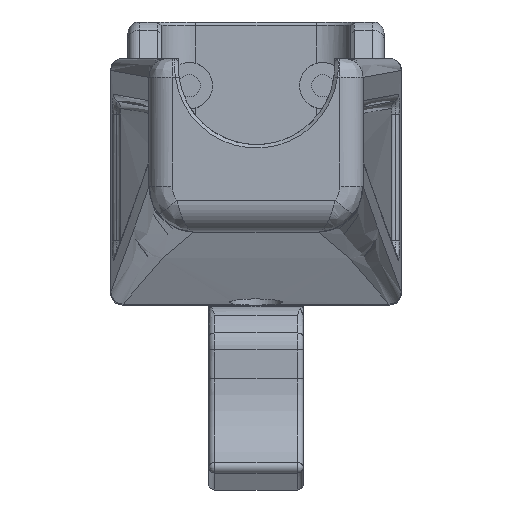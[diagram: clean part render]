
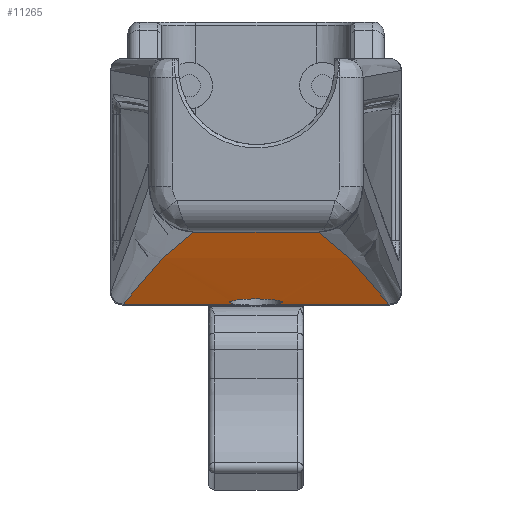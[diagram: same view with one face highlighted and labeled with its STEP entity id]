
A CAD part, front view. The second image highlights one B-rep face of the part: STEP entity #11265.
In plain terms, the highlighted cylindrical face has radius 1594.73 mm (diameter 3189.46 mm), a partial arc.
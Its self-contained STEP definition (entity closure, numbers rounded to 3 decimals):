
#330=B_SPLINE_CURVE_WITH_KNOTS('',3,(#18662,#18663,#18664,#18665,#18666,
#18667,#18668,#18669,#18670,#18671,#18672,#18673,#18674,#18675,#18676,#18677,
#18678,#18679,#18680,#18681,#18682,#18683,#18684),.UNSPECIFIED.,.F.,.F.,
(4,2,2,2,2,2,3,2,2,2,4),(-0.946,-0.852,-0.681,
-0.51,-0.339,-0.169,0.,0.17,
0.34,0.51,0.681),.UNSPECIFIED.);
#332=B_SPLINE_CURVE_WITH_KNOTS('',3,(#18700,#18701,#18702,#18703,#18704,
#18705),.UNSPECIFIED.,.F.,.F.,(4,2,4),(0.681,0.851,
0.946),.UNSPECIFIED.);
#459=B_SPLINE_CURVE_WITH_KNOTS('',3,(#21532,#21533,#21534,#21535),
 .UNSPECIFIED.,.F.,.F.,(4,4),(-0.316,-0.304),
 .UNSPECIFIED.);
#462=B_SPLINE_CURVE_WITH_KNOTS('',3,(#22020,#22021,#22022,#22023),
 .UNSPECIFIED.,.F.,.F.,(4,4),(-15.111,-0.316),
 .UNSPECIFIED.);
#472=B_SPLINE_CURVE_WITH_KNOTS('',3,(#22319,#22320,#22321,#22322),
 .UNSPECIFIED.,.F.,.F.,(4,4),(-0.316,-0.304),
 .UNSPECIFIED.);
#477=B_SPLINE_CURVE_WITH_KNOTS('',3,(#22797,#22798,#22799,#22800),
 .UNSPECIFIED.,.F.,.F.,(4,4),(-15.111,-0.316),
 .UNSPECIFIED.);
#1774=FACE_OUTER_BOUND('',#2480,.T.);
#2480=EDGE_LOOP('',(#9272,#9273,#9274,#9275,#9276,#9277,#9278,#9279,#9280));
#3070=LINE('',#18712,#3874);
#3072=LINE('',#18863,#3876);
#3217=LINE('',#22992,#4021);
#3874=VECTOR('',#13869,10.);
#3876=VECTOR('',#13871,10.);
#4021=VECTOR('',#14404,10.);
#4840=VERTEX_POINT('',#18659);
#4841=VERTEX_POINT('',#18661);
#4842=VERTEX_POINT('',#18685);
#4844=VERTEX_POINT('',#18711);
#4849=VERTEX_POINT('',#18816);
#5079=VERTEX_POINT('',#21518);
#5081=VERTEX_POINT('',#22019);
#5083=VERTEX_POINT('',#22311);
#5085=VERTEX_POINT('',#22788);
#6125=EDGE_CURVE('',#4841,#4840,#330,.T.);
#6127=EDGE_CURVE('',#4840,#4842,#332,.T.);
#6130=EDGE_CURVE('',#4844,#4841,#3070,.T.);
#6136=EDGE_CURVE('',#4842,#4849,#3072,.T.);
#6503=EDGE_CURVE('',#5079,#4844,#459,.T.);
#6506=EDGE_CURVE('',#5081,#5079,#462,.T.);
#6521=EDGE_CURVE('',#5083,#4849,#472,.T.);
#6526=EDGE_CURVE('',#5085,#5083,#477,.T.);
#6533=EDGE_CURVE('',#5085,#5081,#3217,.T.);
#9272=ORIENTED_EDGE('',*,*,#6125,.T.);
#9273=ORIENTED_EDGE('',*,*,#6127,.T.);
#9274=ORIENTED_EDGE('',*,*,#6136,.T.);
#9275=ORIENTED_EDGE('',*,*,#6521,.F.);
#9276=ORIENTED_EDGE('',*,*,#6526,.F.);
#9277=ORIENTED_EDGE('',*,*,#6533,.T.);
#9278=ORIENTED_EDGE('',*,*,#6506,.T.);
#9279=ORIENTED_EDGE('',*,*,#6503,.T.);
#9280=ORIENTED_EDGE('',*,*,#6130,.T.);
#10766=CYLINDRICAL_SURFACE('',#12198,1594.729);
#11265=ADVANCED_FACE('',(#1774),#10766,.F.);
#12198=AXIS2_PLACEMENT_3D('',#22991,#14402,#14403);
#13869=DIRECTION('',(1.,0.,0.));
#13871=DIRECTION('',(1.,0.,0.));
#14402=DIRECTION('center_axis',(-1.,0.,0.));
#14403=DIRECTION('ref_axis',(0.,0.131,0.991));
#14404=DIRECTION('',(-1.,0.,0.));
#18659=CARTESIAN_POINT('',(20.477,-31.891,-156.922));
#18661=CARTESIAN_POINT('',(12.295,-29.303,-157.26));
#18662=CARTESIAN_POINT('Ctrl Pts',(12.295,-29.303,-157.26));
#18663=CARTESIAN_POINT('Ctrl Pts',(12.108,-29.57,-157.225));
#18664=CARTESIAN_POINT('Ctrl Pts',(11.947,-29.861,-157.187));
#18665=CARTESIAN_POINT('Ctrl Pts',(11.59,-30.722,-157.074));
#18666=CARTESIAN_POINT('Ctrl Pts',(11.477,-31.325,-156.995));
#18667=CARTESIAN_POINT('Ctrl Pts',(11.477,-32.456,-156.848));
#18668=CARTESIAN_POINT('Ctrl Pts',(11.59,-33.059,-156.77));
#18669=CARTESIAN_POINT('Ctrl Pts',(12.05,-34.17,-156.627));
#18670=CARTESIAN_POINT('Ctrl Pts',(12.398,-34.677,-156.562));
#18671=CARTESIAN_POINT('Ctrl Pts',(13.198,-35.475,-156.46));
#18672=CARTESIAN_POINT('Ctrl Pts',(13.703,-35.82,-156.416));
#18673=CARTESIAN_POINT('Ctrl Pts',(14.81,-36.278,-156.357));
#18674=CARTESIAN_POINT('Ctrl Pts',(15.412,-36.391,-156.343));
#18675=CARTESIAN_POINT('Ctrl Pts',(15.977,-36.391,-156.343));
#18676=CARTESIAN_POINT('Ctrl Pts',(16.543,-36.391,-156.343));
#18677=CARTESIAN_POINT('Ctrl Pts',(17.146,-36.277,-156.357));
#18678=CARTESIAN_POINT('Ctrl Pts',(18.255,-35.817,-156.416));
#18679=CARTESIAN_POINT('Ctrl Pts',(18.76,-35.471,-156.46));
#18680=CARTESIAN_POINT('Ctrl Pts',(19.559,-34.672,-156.562));
#18681=CARTESIAN_POINT('Ctrl Pts',(19.905,-34.165,-156.627));
#18682=CARTESIAN_POINT('Ctrl Pts',(20.364,-33.057,-156.77));
#18683=CARTESIAN_POINT('Ctrl Pts',(20.477,-32.454,-156.848));
#18684=CARTESIAN_POINT('Ctrl Pts',(20.477,-31.891,-156.922));
#18685=CARTESIAN_POINT('',(19.658,-29.303,-157.26));
#18700=CARTESIAN_POINT('Ctrl Pts',(20.477,-31.891,-156.922));
#18701=CARTESIAN_POINT('Ctrl Pts',(20.477,-31.326,-156.995));
#18702=CARTESIAN_POINT('Ctrl Pts',(20.364,-30.724,-157.074));
#18703=CARTESIAN_POINT('Ctrl Pts',(20.008,-29.863,-157.186));
#18704=CARTESIAN_POINT('Ctrl Pts',(19.846,-29.571,-157.225));
#18705=CARTESIAN_POINT('Ctrl Pts',(19.658,-29.303,-157.26));
#18711=CARTESIAN_POINT('',(-6.934,-29.303,-157.26));
#18712=CARTESIAN_POINT('',(-9.1,-29.303,-157.26));
#18816=CARTESIAN_POINT('',(38.888,-29.303,-157.26));
#18863=CARTESIAN_POINT('',(-9.1,-29.303,-157.26));
#21518=CARTESIAN_POINT('',(-6.923,-29.418,-157.245));
#21532=CARTESIAN_POINT('Ctrl Pts',(-6.923,-29.418,
-157.245));
#21533=CARTESIAN_POINT('Ctrl Pts',(-6.927,-29.38,
-157.25));
#21534=CARTESIAN_POINT('Ctrl Pts',(-6.931,-29.342,
-157.255));
#21535=CARTESIAN_POINT('Ctrl Pts',(-6.934,-29.303,
-157.26));
#22019=CARTESIAN_POINT('',(5.283,-175.713,-144.808));
#22020=CARTESIAN_POINT('Ctrl Pts',(5.283,-175.713,-144.808));
#22021=CARTESIAN_POINT('Ctrl Pts',(2.12,-126.802,-146.705));
#22022=CARTESIAN_POINT('Ctrl Pts',(-1.963,-77.965,
-150.856));
#22023=CARTESIAN_POINT('Ctrl Pts',(-6.923,-29.418,
-157.245));
#22311=CARTESIAN_POINT('',(38.876,-29.418,-157.245));
#22319=CARTESIAN_POINT('Ctrl Pts',(38.876,-29.418,-157.245));
#22320=CARTESIAN_POINT('Ctrl Pts',(38.88,-29.38,-157.25));
#22321=CARTESIAN_POINT('Ctrl Pts',(38.884,-29.342,-157.255));
#22322=CARTESIAN_POINT('Ctrl Pts',(38.888,-29.303,-157.26));
#22788=CARTESIAN_POINT('',(26.67,-175.713,-144.808));
#22797=CARTESIAN_POINT('Ctrl Pts',(26.67,-175.713,-144.808));
#22798=CARTESIAN_POINT('Ctrl Pts',(29.834,-126.802,-146.705));
#22799=CARTESIAN_POINT('Ctrl Pts',(33.916,-77.965,-150.856));
#22800=CARTESIAN_POINT('Ctrl Pts',(38.876,-29.418,-157.245));
#22991=CARTESIAN_POINT('Origin',(41.053,-237.506,-1738.339));
#22992=CARTESIAN_POINT('',(-9.1,-175.713,-144.808));
